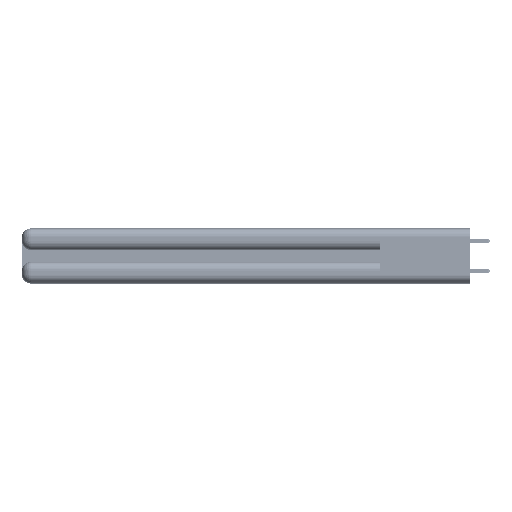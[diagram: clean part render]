
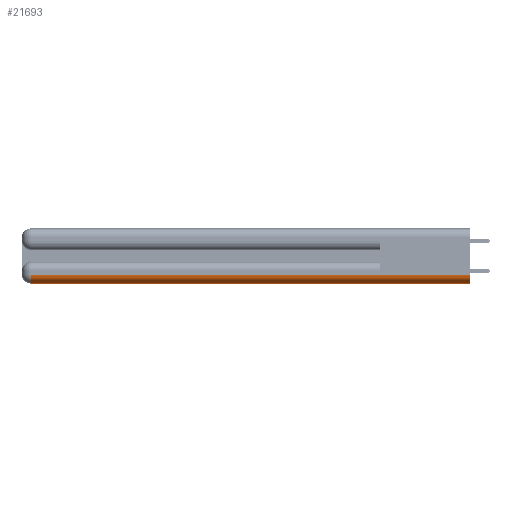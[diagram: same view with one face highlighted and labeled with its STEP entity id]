
A CAD part, left-side view. The second image highlights one B-rep face of the part: STEP entity #21693.
In plain terms, the highlighted cylindrical face has radius 1.524 mm (diameter 3.048 mm), a partial arc.
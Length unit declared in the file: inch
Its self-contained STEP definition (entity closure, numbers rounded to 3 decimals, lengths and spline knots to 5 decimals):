
#769 = AXIS2_PLACEMENT_3D ( 'NONE', #36332, #23937, #44881 ) ;
#2454 = CIRCLE ( 'NONE', #30695, 0.06 ) ;
#3440 = ORIENTED_EDGE ( 'NONE', *, *, #11669, .F. ) ;
#4263 = CARTESIAN_POINT ( 'NONE',  ( 0.06, 3., 0. ) ) ;
#5182 = VERTEX_POINT ( 'NONE', #32005 ) ;
#5385 = CARTESIAN_POINT ( 'NONE',  ( 0.06, 2.94, 0. ) ) ;
#8049 = CARTESIAN_POINT ( 'NONE',  ( 0., 0., 0.06 ) ) ;
#8227 = EDGE_CURVE ( 'NONE', #40229, #22816, #43178, .T. ) ;
#8347 = AXIS2_PLACEMENT_3D ( 'NONE', #53829, #41735, #37468 ) ;
#9089 = ORIENTED_EDGE ( 'NONE', *, *, #8227, .F. ) ;
#11669 = EDGE_CURVE ( 'NONE', #5182, #37224, #53076, .T. ) ;
#15808 = DIRECTION ( 'NONE',  ( 0., 0., 1. ) ) ;
#16407 = DIRECTION ( 'NONE',  ( 0., -1., 0. ) ) ;
#18693 = ORIENTED_EDGE ( 'NONE', *, *, #20422, .F. ) ;
#20422 = EDGE_CURVE ( 'NONE', #37224, #40229, #2454, .T. ) ;
#21303 = VECTOR ( 'NONE', #25872, 39.37008 ) ;
#21693 = ADVANCED_FACE ( 'NONE', ( #22990 ), #37552, .T. ) ;
#22816 = VERTEX_POINT ( 'NONE', #5385 ) ;
#22968 = ORIENTED_EDGE ( 'NONE', *, *, #24664, .F. ) ;
#22990 = FACE_OUTER_BOUND ( 'NONE', #31349, .T. ) ;
#23937 = DIRECTION ( 'NONE',  ( 0., 1., 0. ) ) ;
#24664 = EDGE_CURVE ( 'NONE', #22816, #5182, #43882, .T. ) ;
#25872 = DIRECTION ( 'NONE',  ( 0., 1., 0. ) ) ;
#28862 = CARTESIAN_POINT ( 'NONE',  ( 0., 0., 0.06 ) ) ;
#30695 = AXIS2_PLACEMENT_3D ( 'NONE', #36814, #36626, #15808 ) ;
#31349 = EDGE_LOOP ( 'NONE', ( #18693, #3440, #22968, #9089 ) ) ;
#32005 = CARTESIAN_POINT ( 'NONE',  ( 0., 2.94, 0.06 ) ) ;
#36332 = CARTESIAN_POINT ( 'NONE',  ( 0.06, 0., 0.06 ) ) ;
#36626 = DIRECTION ( 'NONE',  ( 0., -1., 0. ) ) ;
#36814 = CARTESIAN_POINT ( 'NONE',  ( 0.06, 0., 0.06 ) ) ;
#37224 = VERTEX_POINT ( 'NONE', #28862 ) ;
#37468 = DIRECTION ( 'NONE',  ( 0., 0., 1. ) ) ;
#37552 = CYLINDRICAL_SURFACE ( 'NONE', #769, 0.06 ) ;
#38692 = CARTESIAN_POINT ( 'NONE',  ( 0.06, 0., 0. ) ) ;
#40229 = VERTEX_POINT ( 'NONE', #38692 ) ;
#41735 = DIRECTION ( 'NONE',  ( 0., 1., 0. ) ) ;
#43178 = LINE ( 'NONE', #4263, #21303 ) ;
#43882 = CIRCLE ( 'NONE', #8347, 0.06 ) ;
#44881 = DIRECTION ( 'NONE',  ( 0., 0., 1. ) ) ;
#51088 = VECTOR ( 'NONE', #16407, 39.37008 ) ;
#53076 = LINE ( 'NONE', #8049, #51088 ) ;
#53829 = CARTESIAN_POINT ( 'NONE',  ( 0.06, 2.94, 0.06 ) ) ;
